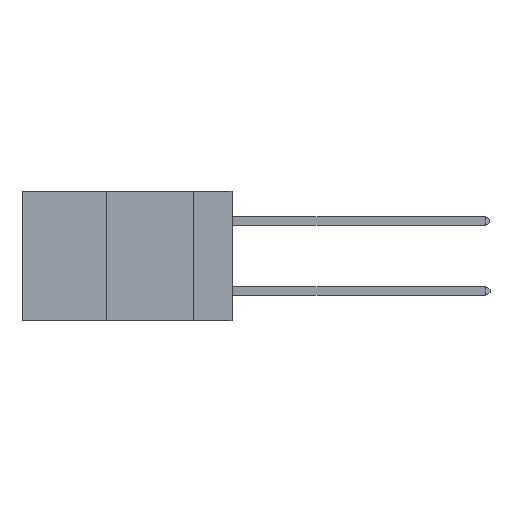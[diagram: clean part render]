
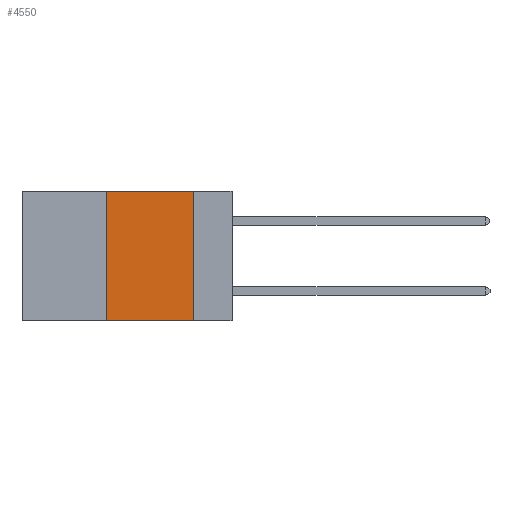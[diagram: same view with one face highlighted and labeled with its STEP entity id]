
A CAD part, left-side view. The second image highlights one B-rep face of the part: STEP entity #4550.
In plain terms, the highlighted planar face has unit normal (-1, 0, 0).
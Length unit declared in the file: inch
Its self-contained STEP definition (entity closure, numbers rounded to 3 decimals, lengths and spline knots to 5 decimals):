
#346 = LINE ( 'NONE', #848, #17339 ) ;
#848 = CARTESIAN_POINT ( 'NONE',  ( 0., 0.11, 0. ) ) ;
#2755 = CARTESIAN_POINT ( 'NONE',  ( 0., 0.36, -0.37 ) ) ;
#2834 = VECTOR ( 'NONE', #13305, 39.37008 ) ;
#3310 = DIRECTION ( 'NONE',  ( 0., -1., 0. ) ) ;
#3470 = CARTESIAN_POINT ( 'NONE',  ( 0., 0.36, 0. ) ) ;
#4550 = ADVANCED_FACE ( 'NONE', ( #12537 ), #14135, .F. ) ;
#5469 = VERTEX_POINT ( 'NONE', #3470 ) ;
#5780 = VECTOR ( 'NONE', #3310, 39.37008 ) ;
#6391 = VERTEX_POINT ( 'NONE', #20265 ) ;
#6422 = VERTEX_POINT ( 'NONE', #2755 ) ;
#6550 = CARTESIAN_POINT ( 'NONE',  ( 0., 0.6, -0.37 ) ) ;
#7227 = EDGE_CURVE ( 'NONE', #5469, #6391, #17276, .T. ) ;
#8050 = VERTEX_POINT ( 'NONE', #9693 ) ;
#8195 = EDGE_LOOP ( 'NONE', ( #15049, #8319, #11417, #15290 ) ) ;
#8319 = ORIENTED_EDGE ( 'NONE', *, *, #7227, .F. ) ;
#9387 = DIRECTION ( 'NONE',  ( 0., 0., -1. ) ) ;
#9693 = CARTESIAN_POINT ( 'NONE',  ( 0., 0.11, -0.37 ) ) ;
#10480 = DIRECTION ( 'NONE',  ( 0., 0., -1. ) ) ;
#10588 = LINE ( 'NONE', #6550, #5780 ) ;
#11403 = LINE ( 'NONE', #16371, #2834 ) ;
#11417 = ORIENTED_EDGE ( 'NONE', *, *, #14776, .F. ) ;
#12195 = EDGE_CURVE ( 'NONE', #6391, #8050, #346, .T. ) ;
#12537 = FACE_OUTER_BOUND ( 'NONE', #8195, .T. ) ;
#12723 = CARTESIAN_POINT ( 'NONE',  ( 0., 0.6, 0. ) ) ;
#13117 = VECTOR ( 'NONE', #17438, 39.37008 ) ;
#13305 = DIRECTION ( 'NONE',  ( 0., 0., 1. ) ) ;
#14135 = PLANE ( 'NONE',  #17925 ) ;
#14776 = EDGE_CURVE ( 'NONE', #6422, #5469, #11403, .T. ) ;
#15049 = ORIENTED_EDGE ( 'NONE', *, *, #12195, .F. ) ;
#15290 = ORIENTED_EDGE ( 'NONE', *, *, #15905, .T. ) ;
#15699 = CARTESIAN_POINT ( 'NONE',  ( 0., 0.6, 0. ) ) ;
#15905 = EDGE_CURVE ( 'NONE', #6422, #8050, #10588, .T. ) ;
#16371 = CARTESIAN_POINT ( 'NONE',  ( 0., 0.36, 0. ) ) ;
#17276 = LINE ( 'NONE', #12723, #13117 ) ;
#17339 = VECTOR ( 'NONE', #10480, 39.37008 ) ;
#17438 = DIRECTION ( 'NONE',  ( 0., -1., 0. ) ) ;
#17925 = AXIS2_PLACEMENT_3D ( 'NONE', #15699, #18842, #9387 ) ;
#18842 = DIRECTION ( 'NONE',  ( 1., 0., 0. ) ) ;
#20265 = CARTESIAN_POINT ( 'NONE',  ( 0., 0.11, 0. ) ) ;
